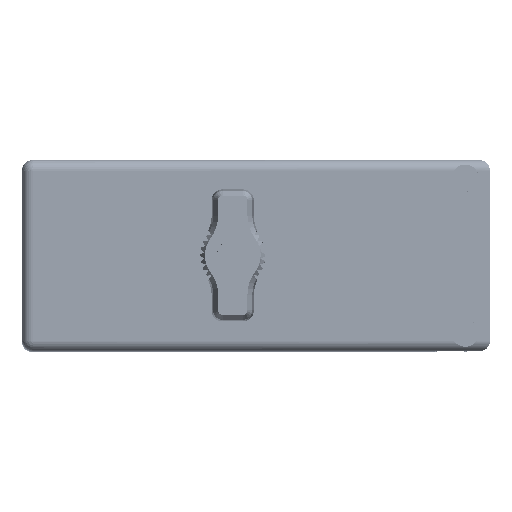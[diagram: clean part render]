
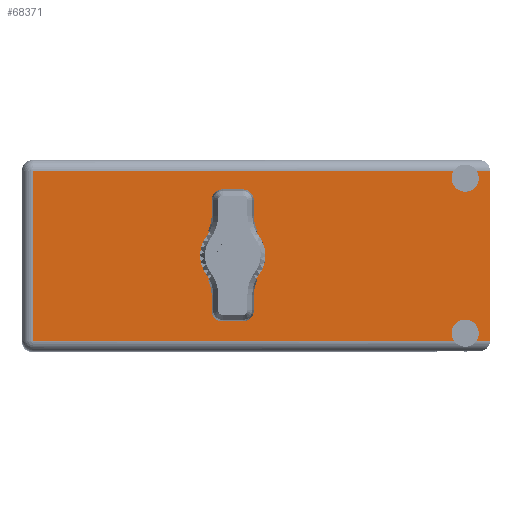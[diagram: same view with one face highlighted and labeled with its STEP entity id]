
A CAD part, top view. The second image highlights one B-rep face of the part: STEP entity #68371.
In plain terms, the highlighted face is planar.
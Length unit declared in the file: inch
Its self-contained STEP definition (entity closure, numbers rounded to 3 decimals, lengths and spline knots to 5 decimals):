
#287 = DIRECTION ( 'NONE',  ( -1., 0., 0. ) ) ;
#2877 = AXIS2_PLACEMENT_3D ( 'NONE', #65472, #80485, #35764 ) ;
#4024 = ORIENTED_EDGE ( 'NONE', *, *, #71650, .F. ) ;
#5657 = DIRECTION ( 'NONE',  ( 0., 1., 0. ) ) ;
#6474 = DIRECTION ( 'NONE',  ( 0., 0., 1. ) ) ;
#6819 = EDGE_LOOP ( 'NONE', ( #76936, #7919, #61294, #26422, #40621, #10473, #35816, #4024, #12679, #66337 ) ) ;
#7919 = ORIENTED_EDGE ( 'NONE', *, *, #33483, .F. ) ;
#8772 = CIRCLE ( 'NONE', #36105, 0.0875 ) ;
#10473 = ORIENTED_EDGE ( 'NONE', *, *, #85682, .T. ) ;
#12082 = EDGE_CURVE ( 'NONE', #65196, #22123, #67189, .T. ) ;
#12679 = ORIENTED_EDGE ( 'NONE', *, *, #88850, .T. ) ;
#14205 = DIRECTION ( 'NONE',  ( 0., 0., 1. ) ) ;
#15931 = DIRECTION ( 'NONE',  ( 0., 1., 0. ) ) ;
#19929 = VERTEX_POINT ( 'NONE', #51849 ) ;
#20022 = CARTESIAN_POINT ( 'NONE',  ( 1.499, 1.675, -0.5 ) ) ;
#20070 = CARTESIAN_POINT ( 'NONE',  ( 0., 1.675, 0. ) ) ;
#20180 = CARTESIAN_POINT ( 'NONE',  ( 1.659, 1.675, 0.547 ) ) ;
#20519 = VERTEX_POINT ( 'NONE', #33061 ) ;
#20623 = VECTOR ( 'NONE', #36113, 39.37008 ) ;
#21275 = VERTEX_POINT ( 'NONE', #20180 ) ;
#22123 = VERTEX_POINT ( 'NONE', #42352 ) ;
#22193 = FACE_BOUND ( 'NONE', #55699, .T. ) ;
#22952 = VERTEX_POINT ( 'NONE', #80709 ) ;
#23456 = CIRCLE ( 'NONE', #2877, 0.125 ) ;
#24067 = VERTEX_POINT ( 'NONE', #79212 ) ;
#26422 = ORIENTED_EDGE ( 'NONE', *, *, #26651, .T. ) ;
#26651 = EDGE_CURVE ( 'NONE', #65196, #21275, #64619, .T. ) ;
#27376 = DIRECTION ( 'NONE',  ( 1., 0., 0. ) ) ;
#27825 = DIRECTION ( 'NONE',  ( 0., 0., 1. ) ) ;
#28208 = DIRECTION ( 'NONE',  ( 0., 1., 0. ) ) ;
#32494 = DIRECTION ( 'NONE',  ( 0., 1., 0. ) ) ;
#33061 = CARTESIAN_POINT ( 'NONE',  ( 1.42519, 1.675, 0.547 ) ) ;
#33483 = EDGE_CURVE ( 'NONE', #22123, #20519, #79274, .T. ) ;
#34860 = VECTOR ( 'NONE', #14205, 39.37008 ) ;
#35764 = DIRECTION ( 'NONE',  ( 0., 0., 1. ) ) ;
#35816 = ORIENTED_EDGE ( 'NONE', *, *, #43199, .F. ) ;
#36105 = AXIS2_PLACEMENT_3D ( 'NONE', #95587, #65864, #6474 ) ;
#36113 = DIRECTION ( 'NONE',  ( 1., 0., 0. ) ) ;
#38112 = CIRCLE ( 'NONE', #95346, 0.0875 ) ;
#38143 = CARTESIAN_POINT ( 'NONE',  ( 1.57281, 1.675, 0.547 ) ) ;
#39297 = LINE ( 'NONE', #51091, #20623 ) ;
#40282 = DIRECTION ( 'NONE',  ( 0., 1., 0. ) ) ;
#40621 = ORIENTED_EDGE ( 'NONE', *, *, #68071, .F. ) ;
#42352 = CARTESIAN_POINT ( 'NONE',  ( 1.499, 1.675, 0.4125 ) ) ;
#43199 = EDGE_CURVE ( 'NONE', #19929, #81333, #8772, .T. ) ;
#46495 = LINE ( 'NONE', #82543, #87332 ) ;
#47499 = CARTESIAN_POINT ( 'NONE',  ( 1.499, 1.675, 0.5 ) ) ;
#47504 = DIRECTION ( 'NONE',  ( 0., 0., 1. ) ) ;
#49040 = ORIENTED_EDGE ( 'NONE', *, *, #87022, .F. ) ;
#49536 = ORIENTED_EDGE ( 'NONE', *, *, #62504, .F. ) ;
#50693 = AXIS2_PLACEMENT_3D ( 'NONE', #80909, #15931, #287 ) ;
#51091 = CARTESIAN_POINT ( 'NONE',  ( 1.659, 1.675, 0.547 ) ) ;
#51411 = CARTESIAN_POINT ( 'NONE',  ( 1.42519, 1.675, -0.547 ) ) ;
#51849 = CARTESIAN_POINT ( 'NONE',  ( 1.499, 1.675, -0.4125 ) ) ;
#53844 = CARTESIAN_POINT ( 'NONE',  ( -1.289, 1.675, -0.547 ) ) ;
#54689 = LINE ( 'NONE', #96736, #34860 ) ;
#55021 = AXIS2_PLACEMENT_3D ( 'NONE', #70324, #32494, #47504 ) ;
#55699 = EDGE_LOOP ( 'NONE', ( #49536, #49040 ) ) ;
#59226 = VERTEX_POINT ( 'NONE', #96288 ) ;
#59497 = EDGE_CURVE ( 'NONE', #78411, #20519, #39297, .T. ) ;
#59514 = FACE_OUTER_BOUND ( 'NONE', #6819, .T. ) ;
#59570 = VERTEX_POINT ( 'NONE', #51411 ) ;
#60147 = CARTESIAN_POINT ( 'NONE',  ( -1.359, 1.675, -0.547 ) ) ;
#60917 = CIRCLE ( 'NONE', #75989, 0.125 ) ;
#61294 = ORIENTED_EDGE ( 'NONE', *, *, #12082, .F. ) ;
#61640 = CARTESIAN_POINT ( 'NONE',  ( -1.289, 1.675, 0.547 ) ) ;
#62206 = VECTOR ( 'NONE', #68332, 39.37008 ) ;
#62504 = EDGE_CURVE ( 'NONE', #59226, #22952, #60917, .T. ) ;
#62826 = DIRECTION ( 'NONE',  ( 0., 0., 1. ) ) ;
#63049 = DIRECTION ( 'NONE',  ( 0., 0., 1. ) ) ;
#64273 = VECTOR ( 'NONE', #63049, 39.37008 ) ;
#64619 = LINE ( 'NONE', #71125, #75064 ) ;
#65196 = VERTEX_POINT ( 'NONE', #38143 ) ;
#65472 = CARTESIAN_POINT ( 'NONE',  ( 0., 1.675, 0. ) ) ;
#65791 = VERTEX_POINT ( 'NONE', #53844 ) ;
#65864 = DIRECTION ( 'NONE',  ( 0., 1., 0. ) ) ;
#66337 = ORIENTED_EDGE ( 'NONE', *, *, #95556, .T. ) ;
#67189 = CIRCLE ( 'NONE', #55021, 0.0875 ) ;
#68071 = EDGE_CURVE ( 'NONE', #24067, #21275, #92249, .T. ) ;
#68332 = DIRECTION ( 'NONE',  ( -1., 0., 0. ) ) ;
#68371 = ADVANCED_FACE ( 'NONE', ( #22193, #59514 ), #81879, .T. ) ;
#70324 = CARTESIAN_POINT ( 'NONE',  ( 1.499, 1.675, 0.5 ) ) ;
#71125 = CARTESIAN_POINT ( 'NONE',  ( 1.659, 1.675, 0.547 ) ) ;
#71650 = EDGE_CURVE ( 'NONE', #59570, #19929, #38112, .T. ) ;
#75064 = VECTOR ( 'NONE', #27376, 39.37008 ) ;
#75989 = AXIS2_PLACEMENT_3D ( 'NONE', #20070, #28208, #95134 ) ;
#76936 = ORIENTED_EDGE ( 'NONE', *, *, #59497, .T. ) ;
#77410 = LINE ( 'NONE', #60147, #62206 ) ;
#78411 = VERTEX_POINT ( 'NONE', #61640 ) ;
#79212 = CARTESIAN_POINT ( 'NONE',  ( 1.659, 1.675, -0.547 ) ) ;
#79274 = CIRCLE ( 'NONE', #82649, 0.0875 ) ;
#80485 = DIRECTION ( 'NONE',  ( 0., 1., 0. ) ) ;
#80709 = CARTESIAN_POINT ( 'NONE',  ( 0., 1.675, -0.125 ) ) ;
#80909 = CARTESIAN_POINT ( 'NONE',  ( -1.359, 1.675, -0.617 ) ) ;
#81333 = VERTEX_POINT ( 'NONE', #95726 ) ;
#81879 = PLANE ( 'NONE',  #50693 ) ;
#82543 = CARTESIAN_POINT ( 'NONE',  ( -1.359, 1.675, -0.547 ) ) ;
#82649 = AXIS2_PLACEMENT_3D ( 'NONE', #47499, #40282, #62826 ) ;
#85682 = EDGE_CURVE ( 'NONE', #24067, #81333, #77410, .T. ) ;
#87022 = EDGE_CURVE ( 'NONE', #22952, #59226, #23456, .T. ) ;
#87332 = VECTOR ( 'NONE', #89065, 39.37008 ) ;
#88850 = EDGE_CURVE ( 'NONE', #59570, #65791, #46495, .T. ) ;
#89065 = DIRECTION ( 'NONE',  ( -1., 0., 0. ) ) ;
#92249 = LINE ( 'NONE', #92722, #64273 ) ;
#92722 = CARTESIAN_POINT ( 'NONE',  ( 1.659, 1.675, 0.617 ) ) ;
#95134 = DIRECTION ( 'NONE',  ( 0., 0., 1. ) ) ;
#95346 = AXIS2_PLACEMENT_3D ( 'NONE', #20022, #5657, #27825 ) ;
#95556 = EDGE_CURVE ( 'NONE', #65791, #78411, #54689, .T. ) ;
#95587 = CARTESIAN_POINT ( 'NONE',  ( 1.499, 1.675, -0.5 ) ) ;
#95726 = CARTESIAN_POINT ( 'NONE',  ( 1.57281, 1.675, -0.547 ) ) ;
#96288 = CARTESIAN_POINT ( 'NONE',  ( 0., 1.675, 0.125 ) ) ;
#96736 = CARTESIAN_POINT ( 'NONE',  ( -1.289, 1.675, -0.617 ) ) ;
